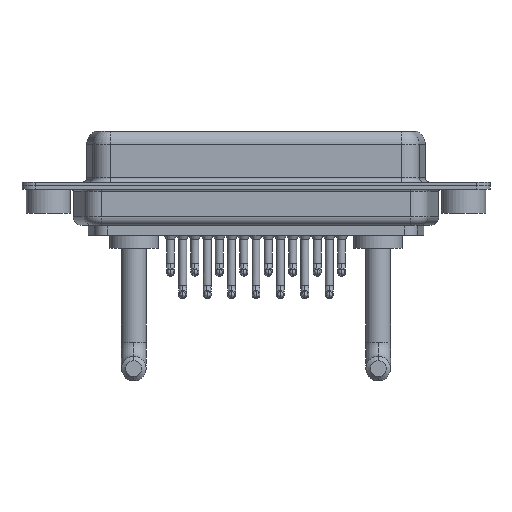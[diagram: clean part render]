
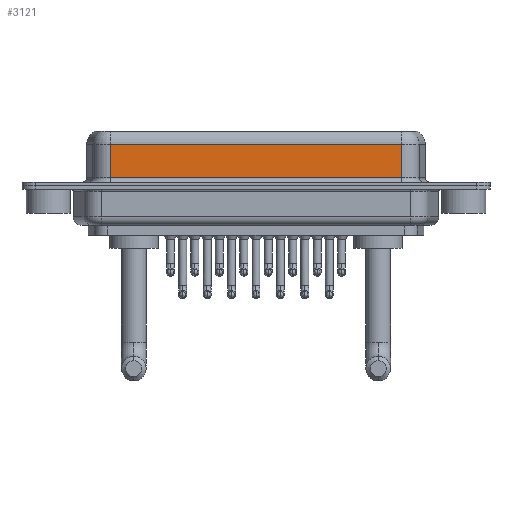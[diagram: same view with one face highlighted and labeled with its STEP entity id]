
A CAD part, front view. The second image highlights one B-rep face of the part: STEP entity #3121.
In plain terms, the highlighted planar face has unit normal (0, -1, 0).
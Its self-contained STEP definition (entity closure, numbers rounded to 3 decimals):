
#806 = ORIENTED_EDGE ( 'NONE', *, *, #12320, .T. ) ;
#2735 = AXIS2_PLACEMENT_3D ( 'NONE', #3475, #9923, #11695 ) ;
#3028 = DIRECTION ( 'NONE',  ( 0., 0., -1. ) ) ;
#3121 = ADVANCED_FACE ( 'NONE', ( #18169 ), #19333, .F. ) ;
#3475 = CARTESIAN_POINT ( 'NONE',  ( 40.037, -3.95, 6.4 ) ) ;
#4367 = CARTESIAN_POINT ( 'NONE',  ( 40.037, -3.95, 4.65 ) ) ;
#4978 = VECTOR ( 'NONE', #3028, 1000. ) ;
#5625 = VERTEX_POINT ( 'NONE', #11470 ) ;
#6094 = LINE ( 'NONE', #17401, #19303 ) ;
#6969 = ORIENTED_EDGE ( 'NONE', *, *, #17760, .T. ) ;
#6975 = EDGE_LOOP ( 'NONE', ( #19763, #6969, #806, #16184 ) ) ;
#8365 = CARTESIAN_POINT ( 'NONE',  ( 40.037, -3.95, 4.65 ) ) ;
#9466 = EDGE_CURVE ( 'NONE', #5625, #11965, #10093, .T. ) ;
#9923 = DIRECTION ( 'NONE',  ( 0., 1., 0. ) ) ;
#10093 = LINE ( 'NONE', #16551, #10817 ) ;
#10299 = VERTEX_POINT ( 'NONE', #4367 ) ;
#10817 = VECTOR ( 'NONE', #19505, 1000. ) ;
#10832 = DIRECTION ( 'NONE',  ( 0., 0., -1. ) ) ;
#11470 = CARTESIAN_POINT ( 'NONE',  ( 7.013, -3.95, 0.9 ) ) ;
#11695 = DIRECTION ( 'NONE',  ( 0., 0., 1. ) ) ;
#11965 = VERTEX_POINT ( 'NONE', #18903 ) ;
#12320 = EDGE_CURVE ( 'NONE', #16245, #5625, #6094, .T. ) ;
#13004 = DIRECTION ( 'NONE',  ( -1., 0., 0. ) ) ;
#13050 = CARTESIAN_POINT ( 'NONE',  ( 7.013, -3.95, 4.65 ) ) ;
#14542 = LINE ( 'NONE', #16146, #4978 ) ;
#16146 = CARTESIAN_POINT ( 'NONE',  ( 40.037, -3.95, 6.4 ) ) ;
#16184 = ORIENTED_EDGE ( 'NONE', *, *, #9466, .T. ) ;
#16245 = VERTEX_POINT ( 'NONE', #13050 ) ;
#16302 = LINE ( 'NONE', #8365, #20105 ) ;
#16551 = CARTESIAN_POINT ( 'NONE',  ( 40.037, -3.95, 0.9 ) ) ;
#17401 = CARTESIAN_POINT ( 'NONE',  ( 7.013, -3.95, 6.4 ) ) ;
#17760 = EDGE_CURVE ( 'NONE', #10299, #16245, #16302, .T. ) ;
#18169 = FACE_OUTER_BOUND ( 'NONE', #6975, .T. ) ;
#18606 = EDGE_CURVE ( 'NONE', #10299, #11965, #14542, .T. ) ;
#18903 = CARTESIAN_POINT ( 'NONE',  ( 40.037, -3.95, 0.9 ) ) ;
#19303 = VECTOR ( 'NONE', #10832, 1000. ) ;
#19333 = PLANE ( 'NONE',  #2735 ) ;
#19505 = DIRECTION ( 'NONE',  ( 1., 0., 0. ) ) ;
#19763 = ORIENTED_EDGE ( 'NONE', *, *, #18606, .F. ) ;
#20105 = VECTOR ( 'NONE', #13004, 1000. ) ;
